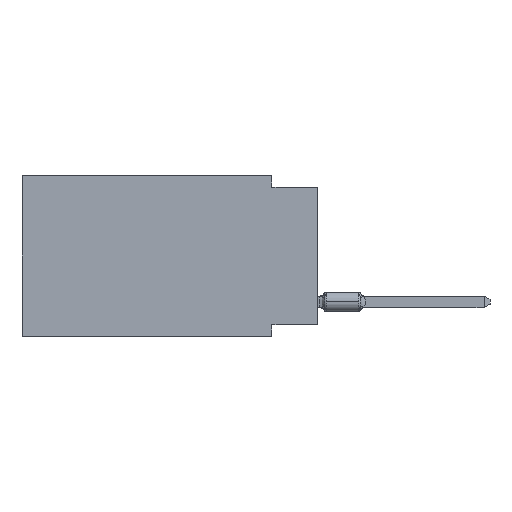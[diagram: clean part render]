
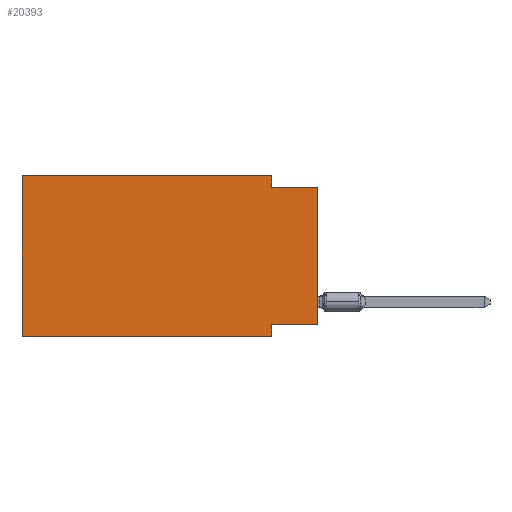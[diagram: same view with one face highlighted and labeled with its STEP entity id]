
A CAD part, left-side view. The second image highlights one B-rep face of the part: STEP entity #20393.
In plain terms, the highlighted planar face has unit normal (-1, 0, 0).
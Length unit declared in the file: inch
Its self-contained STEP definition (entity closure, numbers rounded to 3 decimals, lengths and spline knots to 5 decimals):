
#318 = DIRECTION ( 'NONE',  ( 0., 0., -1. ) ) ;
#729 = VERTEX_POINT ( 'NONE', #30551 ) ;
#896 = ORIENTED_EDGE ( 'NONE', *, *, #18998, .F. ) ;
#1409 = EDGE_CURVE ( 'NONE', #3406, #9417, #11288, .T. ) ;
#1681 = ORIENTED_EDGE ( 'NONE', *, *, #7300, .F. ) ;
#2009 = VECTOR ( 'NONE', #23522, 39.37008 ) ;
#2664 = CARTESIAN_POINT ( 'NONE',  ( 0., 0.645, -0.35 ) ) ;
#3063 = CARTESIAN_POINT ( 'NONE',  ( 0., 0.645, 0. ) ) ;
#3204 = CARTESIAN_POINT ( 'NONE',  ( 0., 0.1, 0. ) ) ;
#3406 = VERTEX_POINT ( 'NONE', #6217 ) ;
#5274 = VERTEX_POINT ( 'NONE', #9048 ) ;
#5819 = PLANE ( 'NONE',  #11150 ) ;
#5951 = CARTESIAN_POINT ( 'NONE',  ( 0., 0., -0.025 ) ) ;
#6217 = CARTESIAN_POINT ( 'NONE',  ( 0., 0.1, 0. ) ) ;
#6288 = CARTESIAN_POINT ( 'NONE',  ( 0., 0.1, -0.35 ) ) ;
#6375 = VECTOR ( 'NONE', #27291, 39.37008 ) ;
#7300 = EDGE_CURVE ( 'NONE', #11642, #18330, #14348, .T. ) ;
#7487 = CARTESIAN_POINT ( 'NONE',  ( 0., 0., -0.325 ) ) ;
#9048 = CARTESIAN_POINT ( 'NONE',  ( 0., 0.645, 0. ) ) ;
#9417 = VERTEX_POINT ( 'NONE', #25643 ) ;
#9879 = CARTESIAN_POINT ( 'NONE',  ( 0., 0., -0.325 ) ) ;
#11150 = AXIS2_PLACEMENT_3D ( 'NONE', #3063, #18120, #318 ) ;
#11288 = LINE ( 'NONE', #3204, #28717 ) ;
#11343 = EDGE_CURVE ( 'NONE', #19920, #28817, #18669, .T. ) ;
#11384 = CARTESIAN_POINT ( 'NONE',  ( 0., 0., 0. ) ) ;
#11642 = VERTEX_POINT ( 'NONE', #25452 ) ;
#13437 = EDGE_LOOP ( 'NONE', ( #26227, #16682, #28028, #17005, #896, #18843, #1681, #31559 ) ) ;
#14348 = LINE ( 'NONE', #26507, #20830 ) ;
#15671 = DIRECTION ( 'NONE',  ( 0., 0., -1. ) ) ;
#16512 = LINE ( 'NONE', #21063, #16517 ) ;
#16517 = VECTOR ( 'NONE', #18630, 39.37008 ) ;
#16682 = ORIENTED_EDGE ( 'NONE', *, *, #26959, .F. ) ;
#16767 = VECTOR ( 'NONE', #17570, 39.37008 ) ;
#16841 = LINE ( 'NONE', #9879, #24635 ) ;
#17005 = ORIENTED_EDGE ( 'NONE', *, *, #28058, .F. ) ;
#17564 = CARTESIAN_POINT ( 'NONE',  ( 0., 0., -0.025 ) ) ;
#17570 = DIRECTION ( 'NONE',  ( 0., -1., 0. ) ) ;
#18055 = CARTESIAN_POINT ( 'NONE',  ( 0., 0.645, 0. ) ) ;
#18120 = DIRECTION ( 'NONE',  ( 1., 0., 0. ) ) ;
#18330 = VERTEX_POINT ( 'NONE', #6288 ) ;
#18630 = DIRECTION ( 'NONE',  ( 0., 0., 1. ) ) ;
#18669 = LINE ( 'NONE', #11384, #2009 ) ;
#18843 = ORIENTED_EDGE ( 'NONE', *, *, #27019, .T. ) ;
#18998 = EDGE_CURVE ( 'NONE', #729, #5274, #16512, .T. ) ;
#19293 = VECTOR ( 'NONE', #24688, 39.37008 ) ;
#19920 = VERTEX_POINT ( 'NONE', #7487 ) ;
#20393 = ADVANCED_FACE ( 'NONE', ( #25253 ), #5819, .F. ) ;
#20830 = VECTOR ( 'NONE', #21791, 39.37008 ) ;
#21063 = CARTESIAN_POINT ( 'NONE',  ( 0., 0.645, 0. ) ) ;
#21577 = EDGE_CURVE ( 'NONE', #19920, #11642, #16841, .T. ) ;
#21791 = DIRECTION ( 'NONE',  ( 0., 0., -1. ) ) ;
#23522 = DIRECTION ( 'NONE',  ( 0., 0., 1. ) ) ;
#24635 = VECTOR ( 'NONE', #30141, 39.37008 ) ;
#24688 = DIRECTION ( 'NONE',  ( 0., -1., 0. ) ) ;
#25253 = FACE_OUTER_BOUND ( 'NONE', #13437, .T. ) ;
#25452 = CARTESIAN_POINT ( 'NONE',  ( 0., 0.1, -0.325 ) ) ;
#25643 = CARTESIAN_POINT ( 'NONE',  ( 0., 0.1, -0.025 ) ) ;
#26227 = ORIENTED_EDGE ( 'NONE', *, *, #11343, .T. ) ;
#26507 = CARTESIAN_POINT ( 'NONE',  ( 0., 0.1, -0.35 ) ) ;
#26959 = EDGE_CURVE ( 'NONE', #9417, #28817, #27123, .T. ) ;
#27019 = EDGE_CURVE ( 'NONE', #729, #18330, #29728, .T. ) ;
#27123 = LINE ( 'NONE', #17564, #19293 ) ;
#27291 = DIRECTION ( 'NONE',  ( 0., -1., 0. ) ) ;
#27938 = LINE ( 'NONE', #18055, #16767 ) ;
#28028 = ORIENTED_EDGE ( 'NONE', *, *, #1409, .F. ) ;
#28058 = EDGE_CURVE ( 'NONE', #5274, #3406, #27938, .T. ) ;
#28717 = VECTOR ( 'NONE', #15671, 39.37008 ) ;
#28817 = VERTEX_POINT ( 'NONE', #5951 ) ;
#29728 = LINE ( 'NONE', #2664, #6375 ) ;
#30141 = DIRECTION ( 'NONE',  ( 0., 1., 0. ) ) ;
#30551 = CARTESIAN_POINT ( 'NONE',  ( 0., 0.645, -0.35 ) ) ;
#31559 = ORIENTED_EDGE ( 'NONE', *, *, #21577, .F. ) ;
